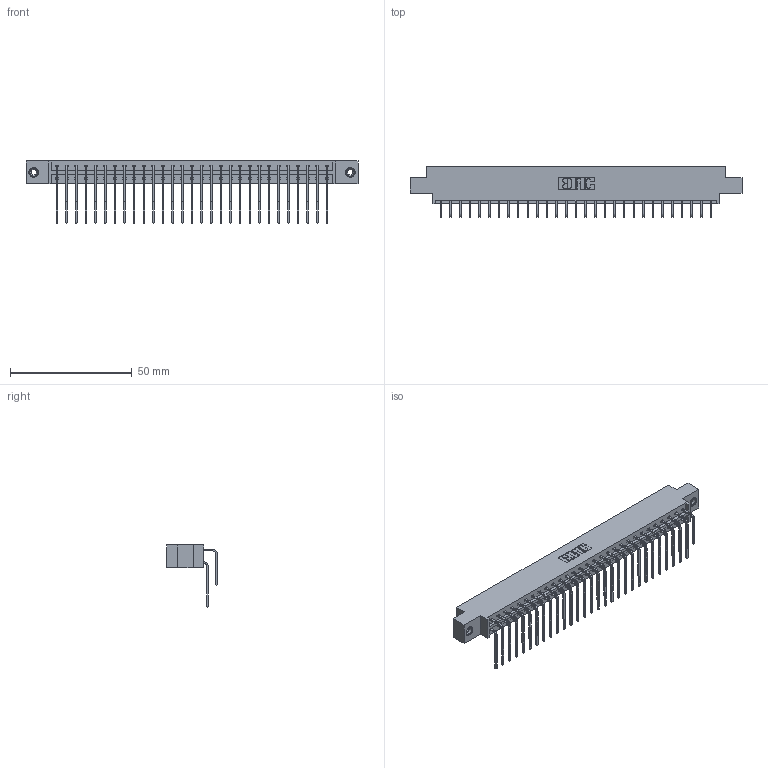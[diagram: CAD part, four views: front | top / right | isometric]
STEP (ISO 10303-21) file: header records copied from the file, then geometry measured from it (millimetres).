
FILE_DESCRIPTION (( 'STEP AP203' ), '1' );
FILE_NAME ('333-058-559-808.STEP', '2018-08-04T06:36:15', ( '' ), ( '' ), 'SwSTEP 2.0', 'SolidWorks 2016', '' );
FILE_SCHEMA (( 'CONFIG_CONTROL_DESIGN' ));
Length unit declared in the file: inch
Products named in the file (5): 333 Part_Offset - .156 Dia - TI; 345-292-001_558 559 Tail - 1; 345-292-001_559 Tail - 2; 345-250-001_345-250-003-102; 333-058-559-808
Assembly tree (61 placements, depth 2):
  333-058-559-808
    333 Part_Offset - .156 Dia - TI
    345-292-001_558 559 Tail - 1  x29
    345-292-001_559 Tail - 2  x29
    345-250-001_345-250-003-102  x2
Bounding box: 136.45 x 20.9 x 25.53 mm (x, y, z)
Volume: 13909.3 mm3; surface area: 18213.8 mm2
Topology: 61 solids, 61 shells, 3310 faces, 9797 edges, 6446 vertices
Faces by surface type: plane 2310, cylinder 984, cone 12, torus 4
Entity records: 23440 total; most frequent: CARTESIAN_POINT 3936, ORIENTED_EDGE 3814, DIRECTION 3397, EDGE_CURVE 1907, VECTOR 1719, LINE 1719, VERTEX_POINT 1264, AXIS2_PLACEMENT_3D 839
